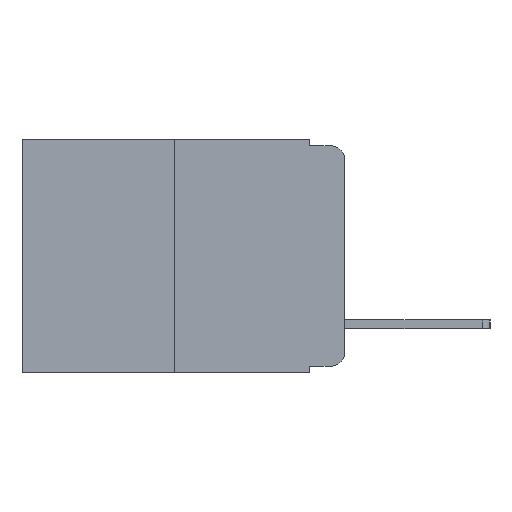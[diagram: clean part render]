
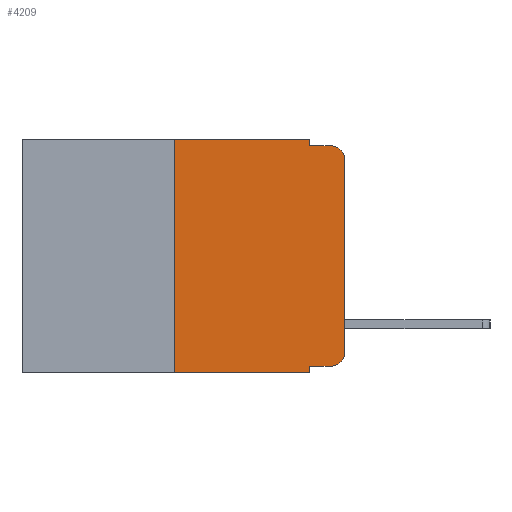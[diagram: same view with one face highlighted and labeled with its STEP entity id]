
A CAD part, left-side view. The second image highlights one B-rep face of the part: STEP entity #4209.
In plain terms, the highlighted planar face has unit normal (-1, 0, 0).
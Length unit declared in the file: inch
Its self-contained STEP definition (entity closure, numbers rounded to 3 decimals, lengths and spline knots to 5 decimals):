
#43 = PLANE ( 'NONE',  #5051 ) ;
#169 = CARTESIAN_POINT ( 'NONE',  ( 0., 0.02, -0.03 ) ) ;
#318 = DIRECTION ( 'NONE',  ( 0., -1., 0. ) ) ;
#697 = EDGE_CURVE ( 'NONE', #4541, #3674, #8989, .T. ) ;
#718 = AXIS2_PLACEMENT_3D ( 'NONE', #169, #7240, #1291 ) ;
#754 = VERTEX_POINT ( 'NONE', #9108 ) ;
#937 = VECTOR ( 'NONE', #318, 39.37008 ) ;
#1130 = CARTESIAN_POINT ( 'NONE',  ( 0., 0.051, -0.01 ) ) ;
#1286 = LINE ( 'NONE', #10177, #937 ) ;
#1291 = DIRECTION ( 'NONE',  ( 0., 0., -1. ) ) ;
#1615 = VECTOR ( 'NONE', #7321, 39.37008 ) ;
#1719 = VERTEX_POINT ( 'NONE', #8283 ) ;
#1896 = VECTOR ( 'NONE', #4450, 39.37008 ) ;
#1916 = LINE ( 'NONE', #6189, #9197 ) ;
#2013 = ORIENTED_EDGE ( 'NONE', *, *, #7926, .F. ) ;
#2073 = AXIS2_PLACEMENT_3D ( 'NONE', #3506, #10216, #4585 ) ;
#2522 = LINE ( 'NONE', #7198, #10014 ) ;
#3151 = ORIENTED_EDGE ( 'NONE', *, *, #7907, .T. ) ;
#3355 = CARTESIAN_POINT ( 'NONE',  ( 0., 0.051, -0.01 ) ) ;
#3400 = VERTEX_POINT ( 'NONE', #10916 ) ;
#3506 = CARTESIAN_POINT ( 'NONE',  ( 0., 0.02, -0.313 ) ) ;
#3674 = VERTEX_POINT ( 'NONE', #10685 ) ;
#3884 = ORIENTED_EDGE ( 'NONE', *, *, #7882, .T. ) ;
#4209 = ADVANCED_FACE ( 'NONE', ( #6416 ), #43, .F. ) ;
#4250 = DIRECTION ( 'NONE',  ( 0., -1., 0. ) ) ;
#4399 = LINE ( 'NONE', #10137, #11526 ) ;
#4450 = DIRECTION ( 'NONE',  ( 0., -1., 0. ) ) ;
#4541 = VERTEX_POINT ( 'NONE', #7175 ) ;
#4585 = DIRECTION ( 'NONE',  ( 0., 0., -1. ) ) ;
#5051 = AXIS2_PLACEMENT_3D ( 'NONE', #8114, #5331, #11798 ) ;
#5318 = CIRCLE ( 'NONE', #718, 0.02 ) ;
#5331 = DIRECTION ( 'NONE',  ( 1., 0., 0. ) ) ;
#5399 = CARTESIAN_POINT ( 'NONE',  ( 0., 0.473, 0. ) ) ;
#5540 = EDGE_LOOP ( 'NONE', ( #3884, #3151, #2013, #11520, #10011, #8472, #8093, #10603, #10749, #6450 ) ) ;
#5625 = CARTESIAN_POINT ( 'NONE',  ( 0., 0.02, -0.01 ) ) ;
#6147 = VECTOR ( 'NONE', #6356, 39.37008 ) ;
#6189 = CARTESIAN_POINT ( 'NONE',  ( 0., 0.473, -0.343 ) ) ;
#6298 = VERTEX_POINT ( 'NONE', #1130 ) ;
#6340 = CIRCLE ( 'NONE', #2073, 0.02 ) ;
#6356 = DIRECTION ( 'NONE',  ( 0., -1., 0. ) ) ;
#6362 = CARTESIAN_POINT ( 'NONE',  ( 0., 0.051, 0. ) ) ;
#6416 = FACE_OUTER_BOUND ( 'NONE', #5540, .T. ) ;
#6450 = ORIENTED_EDGE ( 'NONE', *, *, #8037, .T. ) ;
#6897 = VECTOR ( 'NONE', #8256, 39.37008 ) ;
#6922 = CARTESIAN_POINT ( 'NONE',  ( 0., 0.02, -0.333 ) ) ;
#6993 = EDGE_CURVE ( 'NONE', #3400, #12146, #1916, .T. ) ;
#7175 = CARTESIAN_POINT ( 'NONE',  ( 0., 0.25, 0. ) ) ;
#7198 = CARTESIAN_POINT ( 'NONE',  ( 0., 0., 0. ) ) ;
#7240 = DIRECTION ( 'NONE',  ( -1., 0., 0. ) ) ;
#7302 = CARTESIAN_POINT ( 'NONE',  ( 0., 0., -0.313 ) ) ;
#7321 = DIRECTION ( 'NONE',  ( 0., 0., -1. ) ) ;
#7514 = LINE ( 'NONE', #3355, #1896 ) ;
#7882 = EDGE_CURVE ( 'NONE', #11501, #754, #2522, .T. ) ;
#7907 = EDGE_CURVE ( 'NONE', #754, #10514, #5318, .T. ) ;
#7926 = EDGE_CURVE ( 'NONE', #6298, #10514, #7514, .T. ) ;
#7941 = EDGE_CURVE ( 'NONE', #3674, #6298, #9454, .T. ) ;
#7958 = EDGE_CURVE ( 'NONE', #3400, #4541, #4399, .T. ) ;
#7995 = EDGE_CURVE ( 'NONE', #1719, #12146, #9177, .T. ) ;
#8018 = EDGE_CURVE ( 'NONE', #1719, #9332, #1286, .T. ) ;
#8037 = EDGE_CURVE ( 'NONE', #9332, #11501, #6340, .T. ) ;
#8093 = ORIENTED_EDGE ( 'NONE', *, *, #6993, .T. ) ;
#8114 = CARTESIAN_POINT ( 'NONE',  ( 0., 0.473, 0. ) ) ;
#8179 = DIRECTION ( 'NONE',  ( 0., 0., 1. ) ) ;
#8256 = DIRECTION ( 'NONE',  ( 0., 0., -1. ) ) ;
#8283 = CARTESIAN_POINT ( 'NONE',  ( 0., 0.051, -0.333 ) ) ;
#8301 = CARTESIAN_POINT ( 'NONE',  ( 0., 0.051, 0. ) ) ;
#8472 = ORIENTED_EDGE ( 'NONE', *, *, #7958, .F. ) ;
#8989 = LINE ( 'NONE', #5399, #6147 ) ;
#9108 = CARTESIAN_POINT ( 'NONE',  ( 0., 0., -0.03 ) ) ;
#9177 = LINE ( 'NONE', #8301, #1615 ) ;
#9197 = VECTOR ( 'NONE', #4250, 39.37008 ) ;
#9332 = VERTEX_POINT ( 'NONE', #6922 ) ;
#9454 = LINE ( 'NONE', #6362, #6897 ) ;
#10011 = ORIENTED_EDGE ( 'NONE', *, *, #697, .F. ) ;
#10014 = VECTOR ( 'NONE', #8179, 39.37008 ) ;
#10137 = CARTESIAN_POINT ( 'NONE',  ( 0., 0.25, 0. ) ) ;
#10177 = CARTESIAN_POINT ( 'NONE',  ( 0., 0.051, -0.333 ) ) ;
#10216 = DIRECTION ( 'NONE',  ( -1., 0., 0. ) ) ;
#10514 = VERTEX_POINT ( 'NONE', #5625 ) ;
#10603 = ORIENTED_EDGE ( 'NONE', *, *, #7995, .F. ) ;
#10685 = CARTESIAN_POINT ( 'NONE',  ( 0., 0.051, 0. ) ) ;
#10749 = ORIENTED_EDGE ( 'NONE', *, *, #8018, .T. ) ;
#10916 = CARTESIAN_POINT ( 'NONE',  ( 0., 0.25, -0.343 ) ) ;
#11004 = DIRECTION ( 'NONE',  ( 0., 0., 1. ) ) ;
#11010 = CARTESIAN_POINT ( 'NONE',  ( 0., 0.051, -0.343 ) ) ;
#11501 = VERTEX_POINT ( 'NONE', #7302 ) ;
#11520 = ORIENTED_EDGE ( 'NONE', *, *, #7941, .F. ) ;
#11526 = VECTOR ( 'NONE', #11004, 39.37008 ) ;
#11798 = DIRECTION ( 'NONE',  ( 0., 0., -1. ) ) ;
#12146 = VERTEX_POINT ( 'NONE', #11010 ) ;
